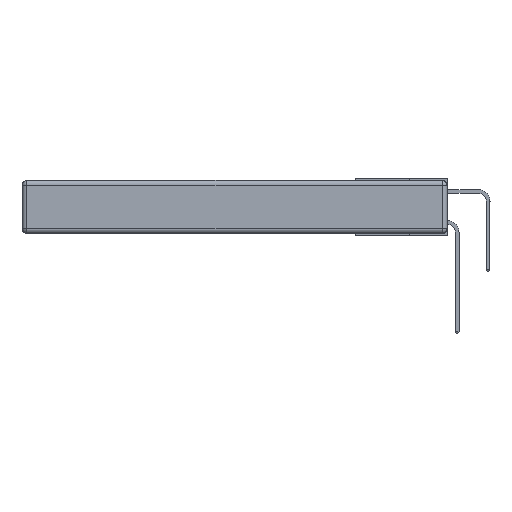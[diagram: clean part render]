
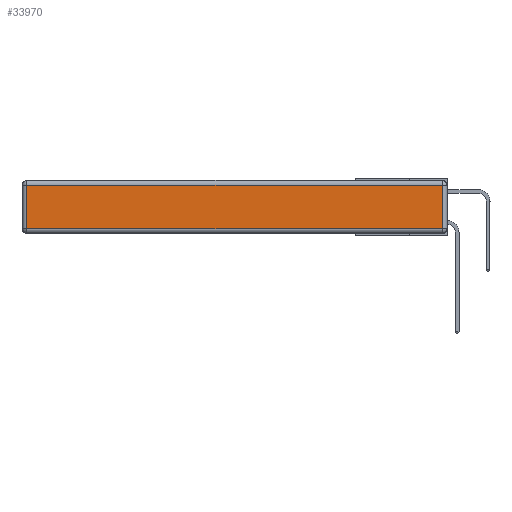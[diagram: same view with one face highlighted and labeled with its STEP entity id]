
A CAD part, left-side view. The second image highlights one B-rep face of the part: STEP entity #33970.
In plain terms, the highlighted planar face has unit normal (-1, 0, 0).
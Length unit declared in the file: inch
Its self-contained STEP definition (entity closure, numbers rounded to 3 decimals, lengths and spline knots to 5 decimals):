
#1797 = ORIENTED_EDGE ( 'NONE', *, *, #36222, .T. ) ;
#2115 = LINE ( 'NONE', #3968, #32142 ) ;
#2585 = CARTESIAN_POINT ( 'NONE',  ( 0., 0., -0.343 ) ) ;
#3968 = CARTESIAN_POINT ( 'NONE',  ( 0., 0.03, -0.343 ) ) ;
#5438 = CARTESIAN_POINT ( 'NONE',  ( 0., 2.72, -0.313 ) ) ;
#5585 = CARTESIAN_POINT ( 'NONE',  ( 0., 0.03, -0.313 ) ) ;
#5917 = LINE ( 'NONE', #26550, #8174 ) ;
#6340 = ORIENTED_EDGE ( 'NONE', *, *, #18076, .T. ) ;
#8043 = LINE ( 'NONE', #37741, #11725 ) ;
#8174 = VECTOR ( 'NONE', #32148, 39.37008 ) ;
#11725 = VECTOR ( 'NONE', #17621, 39.37008 ) ;
#14313 = DIRECTION ( 'NONE',  ( 0., 0., -1. ) ) ;
#14373 = VERTEX_POINT ( 'NONE', #5438 ) ;
#16053 = CARTESIAN_POINT ( 'NONE',  ( 0., 0.03, -0.03 ) ) ;
#16433 = VECTOR ( 'NONE', #14313, 39.37008 ) ;
#17621 = DIRECTION ( 'NONE',  ( 0., -1., 0. ) ) ;
#17802 = EDGE_CURVE ( 'NONE', #14373, #18393, #8043, .T. ) ;
#17925 = CARTESIAN_POINT ( 'NONE',  ( 0., 2.72, -0.03 ) ) ;
#18076 = EDGE_CURVE ( 'NONE', #18393, #33783, #2115, .T. ) ;
#18393 = VERTEX_POINT ( 'NONE', #5585 ) ;
#21563 = EDGE_LOOP ( 'NONE', ( #30305, #6340, #1797, #29112 ) ) ;
#21612 = FACE_OUTER_BOUND ( 'NONE', #21563, .T. ) ;
#21858 = AXIS2_PLACEMENT_3D ( 'NONE', #2585, #22958, #34270 ) ;
#22958 = DIRECTION ( 'NONE',  ( -1., 0., 0. ) ) ;
#26550 = CARTESIAN_POINT ( 'NONE',  ( 0., 2.75, -0.03 ) ) ;
#27720 = VERTEX_POINT ( 'NONE', #17925 ) ;
#29112 = ORIENTED_EDGE ( 'NONE', *, *, #35742, .T. ) ;
#30305 = ORIENTED_EDGE ( 'NONE', *, *, #17802, .T. ) ;
#31402 = LINE ( 'NONE', #34766, #16433 ) ;
#32142 = VECTOR ( 'NONE', #33098, 39.37008 ) ;
#32148 = DIRECTION ( 'NONE',  ( 0., 1., 0. ) ) ;
#33098 = DIRECTION ( 'NONE',  ( 0., 0., 1. ) ) ;
#33783 = VERTEX_POINT ( 'NONE', #16053 ) ;
#33970 = ADVANCED_FACE ( 'NONE', ( #21612 ), #37672, .T. ) ;
#34270 = DIRECTION ( 'NONE',  ( 0., 0., 1. ) ) ;
#34766 = CARTESIAN_POINT ( 'NONE',  ( 0., 2.72, -0.343 ) ) ;
#35742 = EDGE_CURVE ( 'NONE', #27720, #14373, #31402, .T. ) ;
#36222 = EDGE_CURVE ( 'NONE', #33783, #27720, #5917, .T. ) ;
#37672 = PLANE ( 'NONE',  #21858 ) ;
#37741 = CARTESIAN_POINT ( 'NONE',  ( 0., 0., -0.313 ) ) ;
